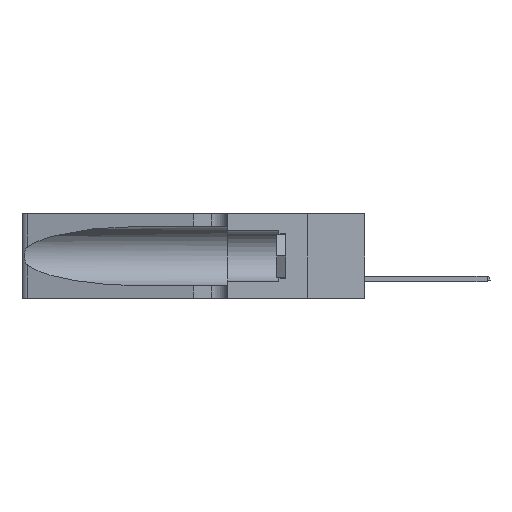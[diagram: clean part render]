
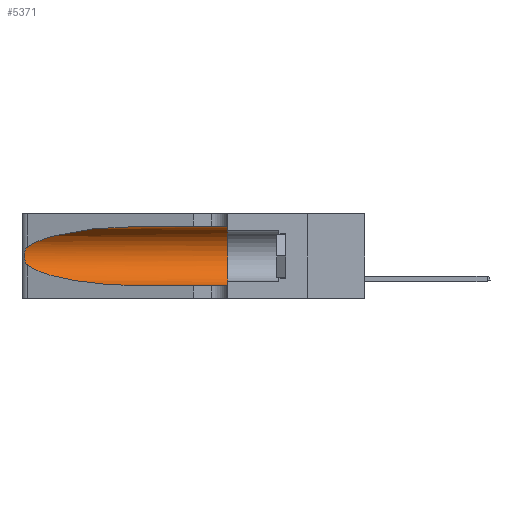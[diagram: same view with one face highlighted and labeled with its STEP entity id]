
A CAD part, left-side view. The second image highlights one B-rep face of the part: STEP entity #5371.
In plain terms, the highlighted cylindrical face has radius 3.308 mm (diameter 6.617 mm), a partial arc.
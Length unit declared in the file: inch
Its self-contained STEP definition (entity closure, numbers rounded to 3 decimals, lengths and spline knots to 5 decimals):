
#762 = CARTESIAN_POINT ( 'NONE',  ( 0.25787, 1.23484, 0.2124 ) ) ;
#1029 = CARTESIAN_POINT ( 'NONE',  ( 0.1305, 1.61858, 0.31525 ) ) ;
#1463 = VERTEX_POINT ( 'NONE', #6665 ) ;
#2858 = CIRCLE ( 'NONE', #5799, 0.13025 ) ;
#3126 = EDGE_CURVE ( 'NONE', #1463, #3853, #44284, .T. ) ;
#3853 = VERTEX_POINT ( 'NONE', #26369 ) ;
#5371 = ADVANCED_FACE ( 'NONE', ( #16344 ), #14688, .F. ) ;
#5799 = AXIS2_PLACEMENT_3D ( 'NONE', #13975, #30891, #17275 ) ;
#6665 = CARTESIAN_POINT ( 'NONE',  ( 0.1305, 0.72297, 0.05475 ) ) ;
#6897 = DIRECTION ( 'NONE',  ( 0., -1., 0. ) ) ;
#7113 = DIRECTION ( 'NONE',  ( 0., 0., -1. ) ) ;
#8706 = CARTESIAN_POINT ( 'NONE',  ( 0.25487, 1.22718, 0.14631 ) ) ;
#9777 = CARTESIAN_POINT ( 'NONE',  ( 0.25487, 1.22718, 0.14631 ) ) ;
#9878 = LINE ( 'NONE', #1029, #36039 ) ;
#11010 = EDGE_LOOP ( 'NONE', ( #39754, #24808, #35019, #34553, #34572, #13619 ) ) ;
#11246 = CARTESIAN_POINT ( 'NONE',  ( 0.25555, 1.22994, 0.2215 ) ) ;
#12918 =( BOUNDED_CURVE ( )  B_SPLINE_CURVE ( 3, ( #30213, #16172, #33013, #22680 ),
 .UNSPECIFIED., .F., .T. ) 
 B_SPLINE_CURVE_WITH_KNOTS ( ( 4, 4 ),
 ( 1.5708, 2.84003 ),
 .UNSPECIFIED. ) 
 CURVE ( )  GEOMETRIC_REPRESENTATION_ITEM ( )  RATIONAL_B_SPLINE_CURVE ( ( 1., 0.87, 0.87, 1. ) ) 
 REPRESENTATION_ITEM ( '' )  );
#13619 = ORIENTED_EDGE ( 'NONE', *, *, #20960, .F. ) ;
#13975 = CARTESIAN_POINT ( 'NONE',  ( 0.1305, 0.35, 0.185 ) ) ;
#14656 = CARTESIAN_POINT ( 'NONE',  ( 0.1305, 0.72297, 0.31525 ) ) ;
#14688 = CYLINDRICAL_SURFACE ( 'NONE', #18048, 0.13025 ) ;
#15270 = CARTESIAN_POINT ( 'NONE',  ( 0.25856, 1.23593, 0.16098 ) ) ;
#15589 = CARTESIAN_POINT ( 'NONE',  ( 0.25639, 1.23186, 0.15144 ) ) ;
#16172 = CARTESIAN_POINT ( 'NONE',  ( 0.18966, 0.96281, 0.31525 ) ) ;
#16344 = FACE_OUTER_BOUND ( 'NONE', #11010, .T. ) ;
#17275 = DIRECTION ( 'NONE',  ( 0., 0., 1. ) ) ;
#17788 = CARTESIAN_POINT ( 'NONE',  ( 0.25487, 1.22718, 0.22369 ) ) ;
#17937 = CARTESIAN_POINT ( 'NONE',  ( 0.25487, 1.22718, 0.22369 ) ) ;
#18048 = AXIS2_PLACEMENT_3D ( 'NONE', #20481, #6897, #7113 ) ;
#18085 = CARTESIAN_POINT ( 'NONE',  ( 0.25854, 1.2359, 0.20912 ) ) ;
#18397 = CARTESIAN_POINT ( 'NONE',  ( 0.25555, 1.22993, 0.14849 ) ) ;
#19758 = CARTESIAN_POINT ( 'NONE',  ( 0.18966, 0.96281, 0.05475 ) ) ;
#20481 = CARTESIAN_POINT ( 'NONE',  ( 0.1305, 1.61858, 0.185 ) ) ;
#20960 = EDGE_CURVE ( 'NONE', #23716, #41423, #9878, .T. ) ;
#22680 = CARTESIAN_POINT ( 'NONE',  ( 0.25487, 1.22718, 0.22369 ) ) ;
#22775 =( BOUNDED_CURVE ( )  B_SPLINE_CURVE ( 3, ( #9777, #33376, #19758, #23202 ),
 .UNSPECIFIED., .F., .F. ) 
 B_SPLINE_CURVE_WITH_KNOTS ( ( 4, 4 ),
 ( 3.44316, 4.71239 ),
 .UNSPECIFIED. ) 
 CURVE ( )  GEOMETRIC_REPRESENTATION_ITEM ( )  RATIONAL_B_SPLINE_CURVE ( ( 1., 0.87, 0.87, 1. ) ) 
 REPRESENTATION_ITEM ( '' )  );
#23202 = CARTESIAN_POINT ( 'NONE',  ( 0.1305, 0.72297, 0.05475 ) ) ;
#23716 = VERTEX_POINT ( 'NONE', #14656 ) ;
#23955 = EDGE_CURVE ( 'NONE', #41423, #3853, #2858, .T. ) ;
#24808 = ORIENTED_EDGE ( 'NONE', *, *, #40004, .T. ) ;
#25022 = DIRECTION ( 'NONE',  ( 0., -1., 0. ) ) ;
#25073 = CARTESIAN_POINT ( 'NONE',  ( 0.26075, 1.23896, 0.178 ) ) ;
#26369 = CARTESIAN_POINT ( 'NONE',  ( 0.1305, 0.35, 0.05475 ) ) ;
#28088 = CARTESIAN_POINT ( 'NONE',  ( 0.25639, 1.23184, 0.21858 ) ) ;
#29174 = CARTESIAN_POINT ( 'NONE',  ( 0.26017, 1.23833, 0.17102 ) ) ;
#30213 = CARTESIAN_POINT ( 'NONE',  ( 0.1305, 0.72297, 0.31525 ) ) ;
#30409 = EDGE_CURVE ( 'NONE', #23716, #33038, #12918, .T. ) ;
#30729 = B_SPLINE_CURVE_WITH_KNOTS ( 'NONE', 3,
 ( #17937, #11246, #28088, #762, #18085, #35301, #42145, #25073, #29174, #15270, #42750, #15589, #18397, #8706 ),
 .UNSPECIFIED., .F., .F.,
 ( 4, 2, 2, 2, 2, 2, 4 ),
 ( 0., 0.00027, 0.00053, 0.00107, 0.0016, 0.00187, 0.00214 ),
 .UNSPECIFIED. ) ;
#30891 = DIRECTION ( 'NONE',  ( 0., 1., 0. ) ) ;
#32295 = DIRECTION ( 'NONE',  ( 0., -1., 0. ) ) ;
#33013 = CARTESIAN_POINT ( 'NONE',  ( 0.2373, 1.15595, 0.28018 ) ) ;
#33038 = VERTEX_POINT ( 'NONE', #17788 ) ;
#33376 = CARTESIAN_POINT ( 'NONE',  ( 0.2373, 1.15595, 0.08982 ) ) ;
#33935 = EDGE_CURVE ( 'NONE', #37244, #1463, #22775, .T. ) ;
#34553 = ORIENTED_EDGE ( 'NONE', *, *, #3126, .T. ) ;
#34572 = ORIENTED_EDGE ( 'NONE', *, *, #23955, .F. ) ;
#34669 = VECTOR ( 'NONE', #32295, 39.37008 ) ;
#35019 = ORIENTED_EDGE ( 'NONE', *, *, #33935, .T. ) ;
#35301 = CARTESIAN_POINT ( 'NONE',  ( 0.26018, 1.23835, 0.19895 ) ) ;
#36039 = VECTOR ( 'NONE', #25022, 39.37008 ) ;
#36207 = CARTESIAN_POINT ( 'NONE',  ( 0.1305, 1.61858, 0.05475 ) ) ;
#36951 = CARTESIAN_POINT ( 'NONE',  ( 0.1305, 0.35, 0.31525 ) ) ;
#37244 = VERTEX_POINT ( 'NONE', #40762 ) ;
#39754 = ORIENTED_EDGE ( 'NONE', *, *, #30409, .T. ) ;
#40004 = EDGE_CURVE ( 'NONE', #33038, #37244, #30729, .T. ) ;
#40762 = CARTESIAN_POINT ( 'NONE',  ( 0.25487, 1.22718, 0.14631 ) ) ;
#41423 = VERTEX_POINT ( 'NONE', #36951 ) ;
#42145 = CARTESIAN_POINT ( 'NONE',  ( 0.26075, 1.23896, 0.19203 ) ) ;
#42750 = CARTESIAN_POINT ( 'NONE',  ( 0.25789, 1.23486, 0.15765 ) ) ;
#44284 = LINE ( 'NONE', #36207, #34669 ) ;
